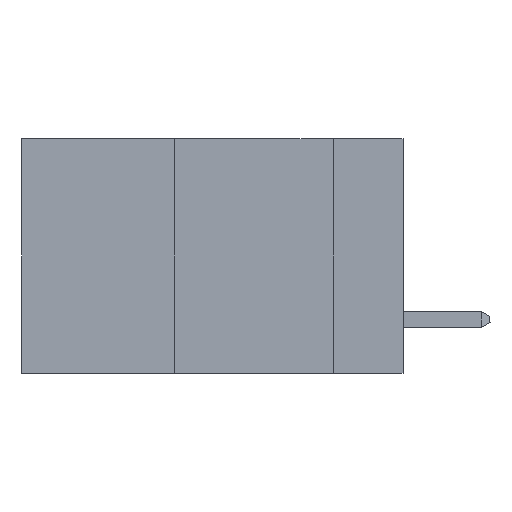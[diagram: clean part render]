
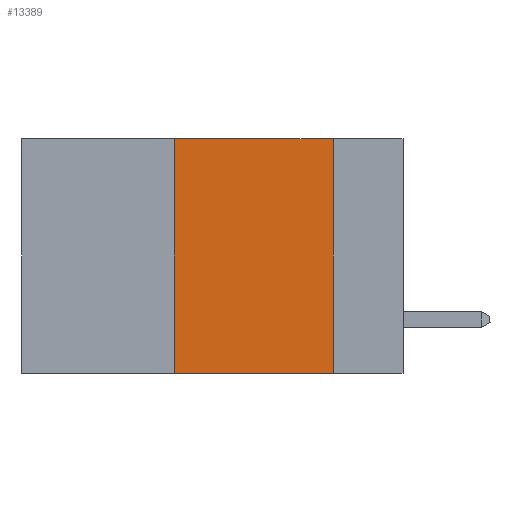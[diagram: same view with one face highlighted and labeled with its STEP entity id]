
A CAD part, left-side view. The second image highlights one B-rep face of the part: STEP entity #13389.
In plain terms, the highlighted planar face has unit normal (-1, 0, 0).
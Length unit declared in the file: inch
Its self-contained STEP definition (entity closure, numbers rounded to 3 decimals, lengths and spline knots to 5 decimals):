
#1608 = CARTESIAN_POINT ( 'NONE',  ( 0., 0.36, 0. ) ) ;
#2011 = DIRECTION ( 'NONE',  ( 1., 0., 0. ) ) ;
#7819 = EDGE_CURVE ( 'NONE', #18768, #38830, #11450, .T. ) ;
#9250 = DIRECTION ( 'NONE',  ( 0., 0., -1. ) ) ;
#9928 = CARTESIAN_POINT ( 'NONE',  ( 0., 0.6, -0.37 ) ) ;
#11450 = LINE ( 'NONE', #22068, #40082 ) ;
#13389 = ADVANCED_FACE ( 'NONE', ( #16355 ), #20324, .F. ) ;
#15773 = DIRECTION ( 'NONE',  ( 0., -1., 0. ) ) ;
#15883 = ORIENTED_EDGE ( 'NONE', *, *, #7819, .F. ) ;
#15887 = ORIENTED_EDGE ( 'NONE', *, *, #32086, .T. ) ;
#16355 = FACE_OUTER_BOUND ( 'NONE', #21501, .T. ) ;
#16656 = CARTESIAN_POINT ( 'NONE',  ( 0., 0.36, -0.37 ) ) ;
#16900 = EDGE_CURVE ( 'NONE', #36184, #27058, #45983, .T. ) ;
#18768 = VERTEX_POINT ( 'NONE', #16656 ) ;
#19566 = VECTOR ( 'NONE', #29802, 39.37008 ) ;
#20165 = CARTESIAN_POINT ( 'NONE',  ( 0., 0.6, 0. ) ) ;
#20246 = CARTESIAN_POINT ( 'NONE',  ( 0., 0.11, 0. ) ) ;
#20324 = PLANE ( 'NONE',  #44262 ) ;
#21501 = EDGE_LOOP ( 'NONE', ( #36396, #33439, #15883, #15887 ) ) ;
#22068 = CARTESIAN_POINT ( 'NONE',  ( 0., 0.36, 0. ) ) ;
#25004 = CARTESIAN_POINT ( 'NONE',  ( 0., 0.11, -0.37 ) ) ;
#25035 = LINE ( 'NONE', #26567, #30260 ) ;
#25112 = CARTESIAN_POINT ( 'NONE',  ( 0., 0.11, 0. ) ) ;
#25826 = DIRECTION ( 'NONE',  ( 0., 0., 1. ) ) ;
#26567 = CARTESIAN_POINT ( 'NONE',  ( 0., 0.6, 0. ) ) ;
#27058 = VERTEX_POINT ( 'NONE', #25004 ) ;
#29802 = DIRECTION ( 'NONE',  ( 0., 0., -1. ) ) ;
#29855 = EDGE_CURVE ( 'NONE', #38830, #36184, #25035, .T. ) ;
#30260 = VECTOR ( 'NONE', #15773, 39.37008 ) ;
#32086 = EDGE_CURVE ( 'NONE', #18768, #27058, #40823, .T. ) ;
#33439 = ORIENTED_EDGE ( 'NONE', *, *, #29855, .F. ) ;
#35734 = DIRECTION ( 'NONE',  ( 0., -1., 0. ) ) ;
#36184 = VERTEX_POINT ( 'NONE', #20246 ) ;
#36396 = ORIENTED_EDGE ( 'NONE', *, *, #16900, .F. ) ;
#37286 = VECTOR ( 'NONE', #35734, 39.37008 ) ;
#38830 = VERTEX_POINT ( 'NONE', #1608 ) ;
#40082 = VECTOR ( 'NONE', #25826, 39.37008 ) ;
#40823 = LINE ( 'NONE', #9928, #37286 ) ;
#44262 = AXIS2_PLACEMENT_3D ( 'NONE', #20165, #2011, #9250 ) ;
#45983 = LINE ( 'NONE', #25112, #19566 ) ;
